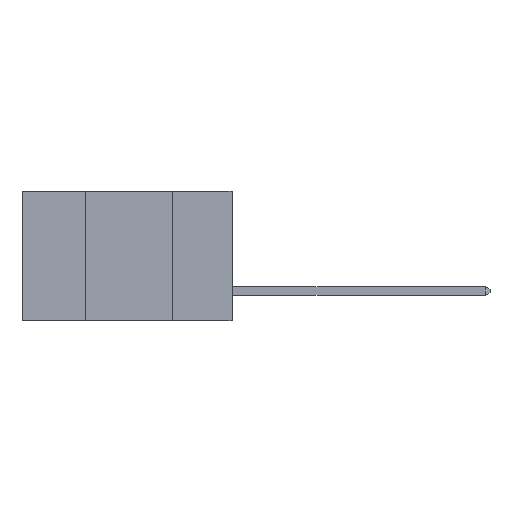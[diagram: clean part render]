
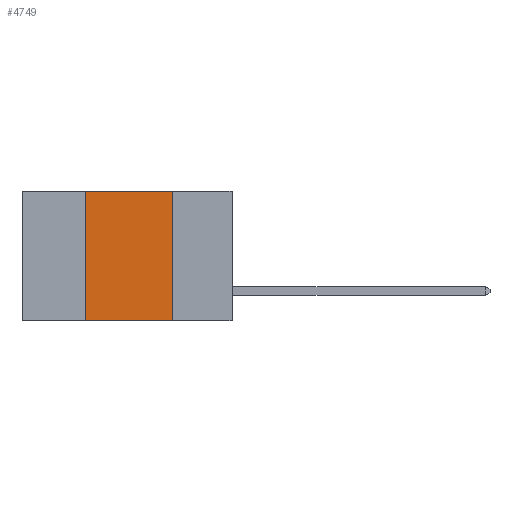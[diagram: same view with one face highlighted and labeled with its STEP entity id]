
A CAD part, left-side view. The second image highlights one B-rep face of the part: STEP entity #4749.
In plain terms, the highlighted planar face has unit normal (-1, 0, 0).
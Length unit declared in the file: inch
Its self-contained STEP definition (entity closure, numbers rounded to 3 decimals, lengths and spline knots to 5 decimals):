
#800 = VECTOR ( 'NONE', #4717, 39.37008 ) ;
#1110 = VERTEX_POINT ( 'NONE', #15291 ) ;
#1862 = EDGE_CURVE ( 'NONE', #2290, #1110, #13624, .T. ) ;
#1912 = EDGE_CURVE ( 'NONE', #10826, #10983, #6932, .T. ) ;
#2290 = VERTEX_POINT ( 'NONE', #9367 ) ;
#3121 = DIRECTION ( 'NONE',  ( 0., -1., 0. ) ) ;
#3480 = CARTESIAN_POINT ( 'NONE',  ( 0., 0.6, 0. ) ) ;
#3599 = EDGE_CURVE ( 'NONE', #2290, #10983, #11422, .T. ) ;
#3838 = ORIENTED_EDGE ( 'NONE', *, *, #1862, .F. ) ;
#4680 = ORIENTED_EDGE ( 'NONE', *, *, #1912, .F. ) ;
#4717 = DIRECTION ( 'NONE',  ( 0., -1., 0. ) ) ;
#4749 = ADVANCED_FACE ( 'NONE', ( #6215 ), #10676, .F. ) ;
#4797 = DIRECTION ( 'NONE',  ( 0., 0., -1. ) ) ;
#6215 = FACE_OUTER_BOUND ( 'NONE', #12272, .T. ) ;
#6574 = DIRECTION ( 'NONE',  ( 1., 0., 0. ) ) ;
#6671 = AXIS2_PLACEMENT_3D ( 'NONE', #12494, #6574, #4797 ) ;
#6932 = LINE ( 'NONE', #14825, #7736 ) ;
#6936 = DIRECTION ( 'NONE',  ( 0., 0., 1. ) ) ;
#7149 = ORIENTED_EDGE ( 'NONE', *, *, #11556, .F. ) ;
#7736 = VECTOR ( 'NONE', #12246, 39.37008 ) ;
#9367 = CARTESIAN_POINT ( 'NONE',  ( 0., 0.42, -0.37 ) ) ;
#9467 = CARTESIAN_POINT ( 'NONE',  ( 0., 0.17, 0. ) ) ;
#9851 = CARTESIAN_POINT ( 'NONE',  ( 0., 0.42, 0. ) ) ;
#10564 = VECTOR ( 'NONE', #6936, 39.37008 ) ;
#10676 = PLANE ( 'NONE',  #6671 ) ;
#10730 = LINE ( 'NONE', #3480, #800 ) ;
#10826 = VERTEX_POINT ( 'NONE', #9467 ) ;
#10983 = VERTEX_POINT ( 'NONE', #14422 ) ;
#11333 = CARTESIAN_POINT ( 'NONE',  ( 0., 0.6, -0.37 ) ) ;
#11422 = LINE ( 'NONE', #11333, #11764 ) ;
#11556 = EDGE_CURVE ( 'NONE', #1110, #10826, #10730, .T. ) ;
#11764 = VECTOR ( 'NONE', #3121, 39.37008 ) ;
#11965 = ORIENTED_EDGE ( 'NONE', *, *, #3599, .T. ) ;
#12246 = DIRECTION ( 'NONE',  ( 0., 0., -1. ) ) ;
#12272 = EDGE_LOOP ( 'NONE', ( #4680, #7149, #3838, #11965 ) ) ;
#12494 = CARTESIAN_POINT ( 'NONE',  ( 0., 0.6, 0. ) ) ;
#13624 = LINE ( 'NONE', #9851, #10564 ) ;
#14422 = CARTESIAN_POINT ( 'NONE',  ( 0., 0.17, -0.37 ) ) ;
#14825 = CARTESIAN_POINT ( 'NONE',  ( 0., 0.17, 0. ) ) ;
#15291 = CARTESIAN_POINT ( 'NONE',  ( 0., 0.42, 0. ) ) ;
